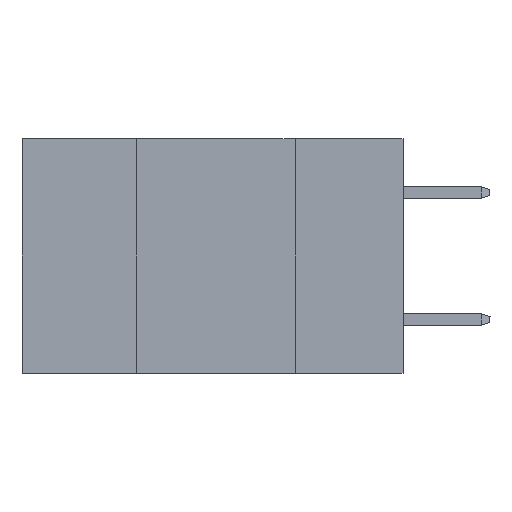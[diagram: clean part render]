
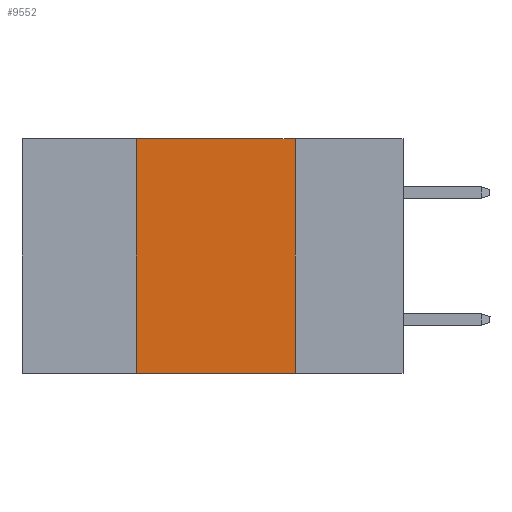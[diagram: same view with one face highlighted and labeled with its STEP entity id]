
A CAD part, left-side view. The second image highlights one B-rep face of the part: STEP entity #9552.
In plain terms, the highlighted planar face has unit normal (-1, 0, 0).
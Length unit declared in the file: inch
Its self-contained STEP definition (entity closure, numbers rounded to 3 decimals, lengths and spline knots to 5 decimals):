
#955 = EDGE_CURVE ( 'NONE', #13409, #8873, #2790, .T. ) ;
#1639 = VERTEX_POINT ( 'NONE', #22728 ) ;
#2790 = LINE ( 'NONE', #3088, #4443 ) ;
#3088 = CARTESIAN_POINT ( 'NONE',  ( 0., 0.6, 0. ) ) ;
#4443 = VECTOR ( 'NONE', #26834, 39.37008 ) ;
#4849 = AXIS2_PLACEMENT_3D ( 'NONE', #26492, #10108, #28968 ) ;
#5139 = VECTOR ( 'NONE', #13203, 39.37008 ) ;
#5976 = VECTOR ( 'NONE', #16787, 39.37008 ) ;
#7395 = LINE ( 'NONE', #16332, #5976 ) ;
#8158 = ORIENTED_EDGE ( 'NONE', *, *, #955, .F. ) ;
#8465 = VERTEX_POINT ( 'NONE', #23464 ) ;
#8873 = VERTEX_POINT ( 'NONE', #21657 ) ;
#9295 = DIRECTION ( 'NONE',  ( 0., 0., -1. ) ) ;
#9552 = ADVANCED_FACE ( 'NONE', ( #15053 ), #12465, .F. ) ;
#10108 = DIRECTION ( 'NONE',  ( 1., 0., 0. ) ) ;
#11116 = EDGE_LOOP ( 'NONE', ( #16685, #8158, #23139, #26069 ) ) ;
#11824 = EDGE_CURVE ( 'NONE', #8465, #1639, #7395, .T. ) ;
#12465 = PLANE ( 'NONE',  #4849 ) ;
#13203 = DIRECTION ( 'NONE',  ( 0., 0., 1. ) ) ;
#13409 = VERTEX_POINT ( 'NONE', #17015 ) ;
#14787 = LINE ( 'NONE', #24192, #5139 ) ;
#15053 = FACE_OUTER_BOUND ( 'NONE', #11116, .T. ) ;
#15921 = CARTESIAN_POINT ( 'NONE',  ( 0., 0.17, 0. ) ) ;
#16332 = CARTESIAN_POINT ( 'NONE',  ( 0., 0.6, -0.37 ) ) ;
#16685 = ORIENTED_EDGE ( 'NONE', *, *, #25752, .F. ) ;
#16787 = DIRECTION ( 'NONE',  ( 0., -1., 0. ) ) ;
#17015 = CARTESIAN_POINT ( 'NONE',  ( 0., 0.42, 0. ) ) ;
#21112 = VECTOR ( 'NONE', #9295, 39.37008 ) ;
#21657 = CARTESIAN_POINT ( 'NONE',  ( 0., 0.17, 0. ) ) ;
#22728 = CARTESIAN_POINT ( 'NONE',  ( 0., 0.17, -0.37 ) ) ;
#23139 = ORIENTED_EDGE ( 'NONE', *, *, #29886, .F. ) ;
#23464 = CARTESIAN_POINT ( 'NONE',  ( 0., 0.42, -0.37 ) ) ;
#24192 = CARTESIAN_POINT ( 'NONE',  ( 0., 0.42, 0. ) ) ;
#25752 = EDGE_CURVE ( 'NONE', #8873, #1639, #27831, .T. ) ;
#26069 = ORIENTED_EDGE ( 'NONE', *, *, #11824, .T. ) ;
#26492 = CARTESIAN_POINT ( 'NONE',  ( 0., 0.6, 0. ) ) ;
#26834 = DIRECTION ( 'NONE',  ( 0., -1., 0. ) ) ;
#27831 = LINE ( 'NONE', #15921, #21112 ) ;
#28968 = DIRECTION ( 'NONE',  ( 0., 0., -1. ) ) ;
#29886 = EDGE_CURVE ( 'NONE', #8465, #13409, #14787, .T. ) ;
